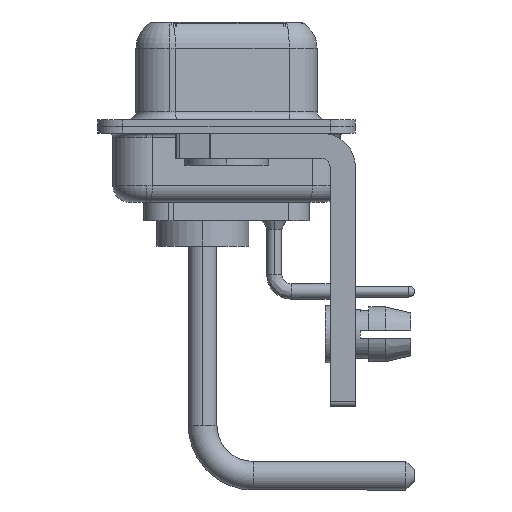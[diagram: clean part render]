
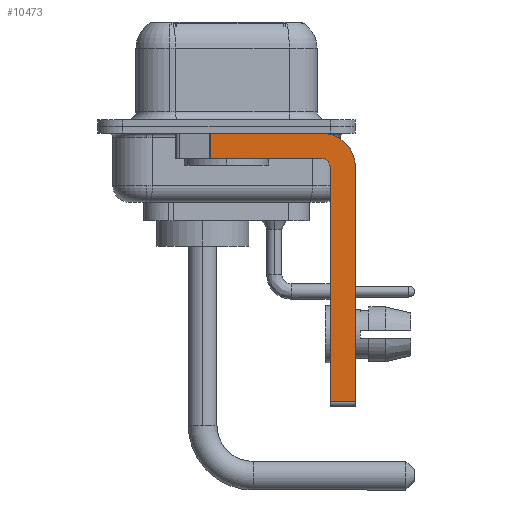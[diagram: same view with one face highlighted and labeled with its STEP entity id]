
A CAD part, left-side view. The second image highlights one B-rep face of the part: STEP entity #10473.
In plain terms, the highlighted planar face has unit normal (-1, 0, 0).
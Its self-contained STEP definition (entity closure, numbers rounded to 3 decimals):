
#199 = VERTEX_POINT ( 'NONE', #15662 ) ;
#220 = LINE ( 'NONE', #9272, #17645 ) ;
#750 = CARTESIAN_POINT ( 'NONE',  ( -2.9, -6.15, -16.6 ) ) ;
#1089 = CARTESIAN_POINT ( 'NONE',  ( -2.9, -5.65, -1.9 ) ) ;
#1783 = CARTESIAN_POINT ( 'NONE',  ( -2.9, -5.65, -0.4 ) ) ;
#1804 = VERTEX_POINT ( 'NONE', #20242 ) ;
#1987 = ORIENTED_EDGE ( 'NONE', *, *, #7131, .T. ) ;
#3040 = EDGE_CURVE ( 'NONE', #199, #17245, #11603, .T. ) ;
#3697 = VECTOR ( 'NONE', #17077, 1000. ) ;
#4038 = DIRECTION ( 'NONE',  ( 0., -1., 0. ) ) ;
#4576 = DIRECTION ( 'NONE',  ( 0., -1., 0. ) ) ;
#4790 = CARTESIAN_POINT ( 'NONE',  ( -2.9, -7.65, -2.4 ) ) ;
#4974 = ORIENTED_EDGE ( 'NONE', *, *, #8533, .F. ) ;
#5273 = EDGE_CURVE ( 'NONE', #17245, #8895, #7505, .T. ) ;
#5892 = FACE_OUTER_BOUND ( 'NONE', #6887, .T. ) ;
#6044 = EDGE_CURVE ( 'NONE', #10215, #199, #10034, .T. ) ;
#6350 = EDGE_CURVE ( 'NONE', #7954, #15756, #20133, .T. ) ;
#6887 = EDGE_LOOP ( 'NONE', ( #11120, #15150, #8399, #15550, #8471, #1987, #4974, #16750 ) ) ;
#7079 = CARTESIAN_POINT ( 'NONE',  ( -2.9, -7.65, -16.35 ) ) ;
#7131 = EDGE_CURVE ( 'NONE', #10215, #16741, #20909, .T. ) ;
#7187 = CARTESIAN_POINT ( 'NONE',  ( -2.9, 0.978, -1.9 ) ) ;
#7214 = CARTESIAN_POINT ( 'NONE',  ( -2.9, -6.15, -16.35 ) ) ;
#7452 = PLANE ( 'NONE',  #19435 ) ;
#7505 = LINE ( 'NONE', #10824, #12013 ) ;
#7954 = VERTEX_POINT ( 'NONE', #1783 ) ;
#8399 = ORIENTED_EDGE ( 'NONE', *, *, #5273, .F. ) ;
#8471 = ORIENTED_EDGE ( 'NONE', *, *, #6044, .F. ) ;
#8533 = EDGE_CURVE ( 'NONE', #15756, #16741, #9250, .T. ) ;
#8673 = EDGE_CURVE ( 'NONE', #1804, #8895, #11502, .T. ) ;
#8895 = VERTEX_POINT ( 'NONE', #7187 ) ;
#9250 = LINE ( 'NONE', #11140, #23322 ) ;
#9272 = CARTESIAN_POINT ( 'NONE',  ( -2.9, 3., -0.4 ) ) ;
#9423 = CARTESIAN_POINT ( 'NONE',  ( -2.9, -5.65, -2.4 ) ) ;
#9459 = DIRECTION ( 'NONE',  ( 0., 0., -1. ) ) ;
#10034 = LINE ( 'NONE', #750, #3697 ) ;
#10215 = VERTEX_POINT ( 'NONE', #7214 ) ;
#10473 = ADVANCED_FACE ( 'NONE', ( #5892 ), #7452, .F. ) ;
#10824 = CARTESIAN_POINT ( 'NONE',  ( -2.9, -5.65, -1.9 ) ) ;
#11120 = ORIENTED_EDGE ( 'NONE', *, *, #13132, .F. ) ;
#11140 = CARTESIAN_POINT ( 'NONE',  ( -2.9, -7.65, -2.4 ) ) ;
#11356 = DIRECTION ( 'NONE',  ( 1., 0., 0. ) ) ;
#11480 = CARTESIAN_POINT ( 'NONE',  ( -2.9, -5.65, -2.4 ) ) ;
#11502 = LINE ( 'NONE', #22157, #14126 ) ;
#11603 = CIRCLE ( 'NONE', #15053, 0.5 ) ;
#12013 = VECTOR ( 'NONE', #18121, 1000. ) ;
#12417 = CARTESIAN_POINT ( 'NONE',  ( -2.9, -5.65, -2.4 ) ) ;
#12820 = DIRECTION ( 'NONE',  ( 0., 0., -1. ) ) ;
#12882 = AXIS2_PLACEMENT_3D ( 'NONE', #9423, #22455, #16823 ) ;
#13132 = EDGE_CURVE ( 'NONE', #1804, #7954, #220, .T. ) ;
#14126 = VECTOR ( 'NONE', #17916, 1000. ) ;
#14319 = DIRECTION ( 'NONE',  ( -1., 0., 0. ) ) ;
#15053 = AXIS2_PLACEMENT_3D ( 'NONE', #12417, #14319, #22959 ) ;
#15150 = ORIENTED_EDGE ( 'NONE', *, *, #8673, .T. ) ;
#15414 = CARTESIAN_POINT ( 'NONE',  ( -2.9, -5.65, -16.35 ) ) ;
#15550 = ORIENTED_EDGE ( 'NONE', *, *, #3040, .F. ) ;
#15662 = CARTESIAN_POINT ( 'NONE',  ( -2.9, -6.15, -2.4 ) ) ;
#15756 = VERTEX_POINT ( 'NONE', #4790 ) ;
#16741 = VERTEX_POINT ( 'NONE', #7079 ) ;
#16750 = ORIENTED_EDGE ( 'NONE', *, *, #6350, .F. ) ;
#16823 = DIRECTION ( 'NONE',  ( 0., 0., -1. ) ) ;
#17077 = DIRECTION ( 'NONE',  ( 0., 0., 1. ) ) ;
#17245 = VERTEX_POINT ( 'NONE', #1089 ) ;
#17645 = VECTOR ( 'NONE', #4038, 1000. ) ;
#17916 = DIRECTION ( 'NONE',  ( 0., 0., -1. ) ) ;
#18121 = DIRECTION ( 'NONE',  ( 0., 1., 0. ) ) ;
#19435 = AXIS2_PLACEMENT_3D ( 'NONE', #11480, #11356, #9459 ) ;
#20133 = CIRCLE ( 'NONE', #12882, 2. ) ;
#20242 = CARTESIAN_POINT ( 'NONE',  ( -2.9, 0.978, -0.4 ) ) ;
#20909 = LINE ( 'NONE', #15414, #22483 ) ;
#22157 = CARTESIAN_POINT ( 'NONE',  ( -2.9, 0.978, -1.9 ) ) ;
#22455 = DIRECTION ( 'NONE',  ( 1., 0., 0. ) ) ;
#22483 = VECTOR ( 'NONE', #4576, 1000. ) ;
#22959 = DIRECTION ( 'NONE',  ( 0., 0., 1. ) ) ;
#23322 = VECTOR ( 'NONE', #12820, 1000. ) ;
